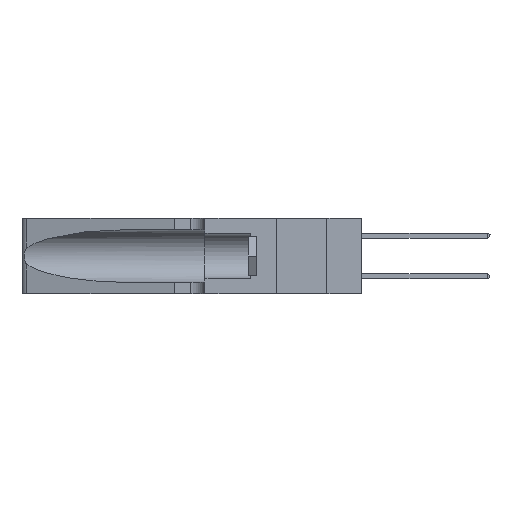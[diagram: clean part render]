
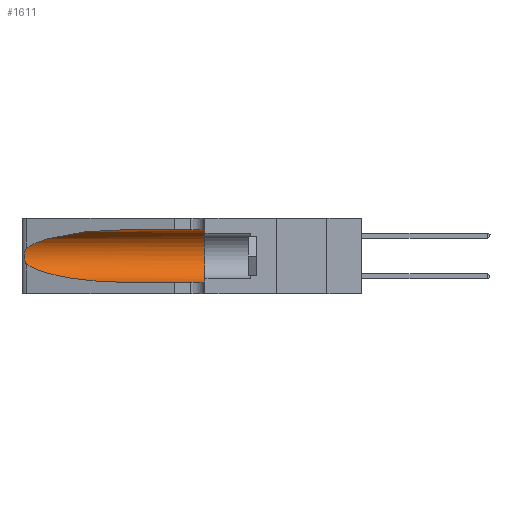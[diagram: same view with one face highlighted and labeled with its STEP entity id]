
A CAD part, left-side view. The second image highlights one B-rep face of the part: STEP entity #1611.
In plain terms, the highlighted cylindrical face has radius 3.308 mm (diameter 6.617 mm), a partial arc.
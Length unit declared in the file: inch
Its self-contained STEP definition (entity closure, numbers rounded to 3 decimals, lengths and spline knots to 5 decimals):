
#44 = CARTESIAN_POINT ( 'NONE',  ( 0.25787, 1.23484, 0.2124 ) ) ;
#296 = ORIENTED_EDGE ( 'NONE', *, *, #22079, .T. ) ;
#915 = DIRECTION ( 'NONE',  ( 0., -1., 0. ) ) ;
#1149 = VECTOR ( 'NONE', #2355, 39.37008 ) ;
#1187 = EDGE_CURVE ( 'NONE', #2431, #9697, #15018, .T. ) ;
#1225 = EDGE_LOOP ( 'NONE', ( #23990, #16633, #296, #6684, #9184, #4881 ) ) ;
#1360 = CARTESIAN_POINT ( 'NONE',  ( 0.25487, 1.22718, 0.22369 ) ) ;
#1387 = CARTESIAN_POINT ( 'NONE',  ( 0.2373, 1.15595, 0.28018 ) ) ;
#1611 = ADVANCED_FACE ( 'NONE', ( #5972 ), #9852, .F. ) ;
#1834 = B_SPLINE_CURVE_WITH_KNOTS ( 'NONE', 3,
 ( #7673, #3776, #11485, #44, #13356, #1963, #15189, #3865, #17033, #5802, #18868, #7752, #20714, #9644 ),
 .UNSPECIFIED., .F., .F.,
 ( 4, 2, 2, 2, 2, 2, 4 ),
 ( 0., 0.00027, 0.00053, 0.00107, 0.0016, 0.00187, 0.00214 ),
 .UNSPECIFIED. ) ;
#1963 = CARTESIAN_POINT ( 'NONE',  ( 0.26018, 1.23835, 0.19895 ) ) ;
#2355 = DIRECTION ( 'NONE',  ( 0., -1., 0. ) ) ;
#2431 = VERTEX_POINT ( 'NONE', #19040 ) ;
#2744 = CARTESIAN_POINT ( 'NONE',  ( 0.1305, 1.61858, 0.05475 ) ) ;
#2978 = CARTESIAN_POINT ( 'NONE',  ( 0.1305, 0.72297, 0.31525 ) ) ;
#3038 = CARTESIAN_POINT ( 'NONE',  ( 0.18966, 0.96281, 0.31525 ) ) ;
#3776 = CARTESIAN_POINT ( 'NONE',  ( 0.25555, 1.22994, 0.2215 ) ) ;
#3821 = LINE ( 'NONE', #2744, #23099 ) ;
#3851 = VERTEX_POINT ( 'NONE', #4462 ) ;
#3865 = CARTESIAN_POINT ( 'NONE',  ( 0.26075, 1.23896, 0.178 ) ) ;
#4462 = CARTESIAN_POINT ( 'NONE',  ( 0.1305, 0.72297, 0.05475 ) ) ;
#4510 = EDGE_CURVE ( 'NONE', #13947, #12311, #17577, .T. ) ;
#4881 = ORIENTED_EDGE ( 'NONE', *, *, #21112, .F. ) ;
#5622 = LINE ( 'NONE', #8138, #1149 ) ;
#5802 = CARTESIAN_POINT ( 'NONE',  ( 0.25856, 1.23593, 0.16098 ) ) ;
#5972 = FACE_OUTER_BOUND ( 'NONE', #1225, .T. ) ;
#6684 = ORIENTED_EDGE ( 'NONE', *, *, #17237, .T. ) ;
#7355 = CARTESIAN_POINT ( 'NONE',  ( 0.2373, 1.15595, 0.08982 ) ) ;
#7673 = CARTESIAN_POINT ( 'NONE',  ( 0.25487, 1.22718, 0.22369 ) ) ;
#7752 = CARTESIAN_POINT ( 'NONE',  ( 0.25639, 1.23186, 0.15144 ) ) ;
#8138 = CARTESIAN_POINT ( 'NONE',  ( 0.1305, 1.61858, 0.31525 ) ) ;
#8910 = CARTESIAN_POINT ( 'NONE',  ( 0.25487, 1.22718, 0.22369 ) ) ;
#9184 = ORIENTED_EDGE ( 'NONE', *, *, #4510, .F. ) ;
#9644 = CARTESIAN_POINT ( 'NONE',  ( 0.25487, 1.22718, 0.14631 ) ) ;
#9697 = VERTEX_POINT ( 'NONE', #8910 ) ;
#9833 = CARTESIAN_POINT ( 'NONE',  ( 0.1305, 0.35, 0.31525 ) ) ;
#9852 = CYLINDRICAL_SURFACE ( 'NONE', #22657, 0.13025 ) ;
#10063 = DIRECTION ( 'NONE',  ( 0., 1., 0. ) ) ;
#11485 = CARTESIAN_POINT ( 'NONE',  ( 0.25639, 1.23184, 0.21858 ) ) ;
#11502 = CARTESIAN_POINT ( 'NONE',  ( 0.1305, 0.72297, 0.05475 ) ) ;
#11970 = CARTESIAN_POINT ( 'NONE',  ( 0.1305, 0.35, 0.05475 ) ) ;
#12139 = EDGE_CURVE ( 'NONE', #9697, #14757, #1834, .T. ) ;
#12311 = VERTEX_POINT ( 'NONE', #11970 ) ;
#12968 = CARTESIAN_POINT ( 'NONE',  ( 0.25487, 1.22718, 0.14631 ) ) ;
#13356 = CARTESIAN_POINT ( 'NONE',  ( 0.25854, 1.2359, 0.20912 ) ) ;
#13947 = VERTEX_POINT ( 'NONE', #9833 ) ;
#14757 = VERTEX_POINT ( 'NONE', #15798 ) ;
#15018 =( BOUNDED_CURVE ( )  B_SPLINE_CURVE ( 3, ( #2978, #3038, #1387, #1360 ),
 .UNSPECIFIED., .F., .F. ) 
 B_SPLINE_CURVE_WITH_KNOTS ( ( 4, 4 ),
 ( 1.5708, 2.84003 ),
 .UNSPECIFIED. ) 
 CURVE ( )  GEOMETRIC_REPRESENTATION_ITEM ( )  RATIONAL_B_SPLINE_CURVE ( ( 1., 0.87, 0.87, 1. ) ) 
 REPRESENTATION_ITEM ( '' )  );
#15189 = CARTESIAN_POINT ( 'NONE',  ( 0.26075, 1.23896, 0.19203 ) ) ;
#15798 = CARTESIAN_POINT ( 'NONE',  ( 0.25487, 1.22718, 0.14631 ) ) ;
#16633 = ORIENTED_EDGE ( 'NONE', *, *, #12139, .T. ) ;
#17033 = CARTESIAN_POINT ( 'NONE',  ( 0.26017, 1.23833, 0.17102 ) ) ;
#17236 = DIRECTION ( 'NONE',  ( 0., -1., 0. ) ) ;
#17237 = EDGE_CURVE ( 'NONE', #3851, #12311, #3821, .T. ) ;
#17291 = DIRECTION ( 'NONE',  ( 0., 0., -1. ) ) ;
#17497 = CARTESIAN_POINT ( 'NONE',  ( 0.1305, 1.61858, 0.185 ) ) ;
#17577 = CIRCLE ( 'NONE', #17609, 0.13025 ) ;
#17609 = AXIS2_PLACEMENT_3D ( 'NONE', #21134, #10063, #22965 ) ;
#18868 = CARTESIAN_POINT ( 'NONE',  ( 0.25789, 1.23486, 0.15765 ) ) ;
#19040 = CARTESIAN_POINT ( 'NONE',  ( 0.1305, 0.72297, 0.31525 ) ) ;
#20007 =( BOUNDED_CURVE ( )  B_SPLINE_CURVE ( 3, ( #12968, #7355, #22496, #11502 ),
 .UNSPECIFIED., .F., .T. ) 
 B_SPLINE_CURVE_WITH_KNOTS ( ( 4, 4 ),
 ( 3.44316, 4.71239 ),
 .UNSPECIFIED. ) 
 CURVE ( )  GEOMETRIC_REPRESENTATION_ITEM ( )  RATIONAL_B_SPLINE_CURVE ( ( 1., 0.87, 0.87, 1. ) ) 
 REPRESENTATION_ITEM ( '' )  );
#20714 = CARTESIAN_POINT ( 'NONE',  ( 0.25555, 1.22993, 0.14849 ) ) ;
#21112 = EDGE_CURVE ( 'NONE', #2431, #13947, #5622, .T. ) ;
#21134 = CARTESIAN_POINT ( 'NONE',  ( 0.1305, 0.35, 0.185 ) ) ;
#22079 = EDGE_CURVE ( 'NONE', #14757, #3851, #20007, .T. ) ;
#22496 = CARTESIAN_POINT ( 'NONE',  ( 0.18966, 0.96281, 0.05475 ) ) ;
#22657 = AXIS2_PLACEMENT_3D ( 'NONE', #17497, #17236, #17291 ) ;
#22965 = DIRECTION ( 'NONE',  ( 0., 0., 1. ) ) ;
#23099 = VECTOR ( 'NONE', #915, 39.37008 ) ;
#23990 = ORIENTED_EDGE ( 'NONE', *, *, #1187, .T. ) ;
